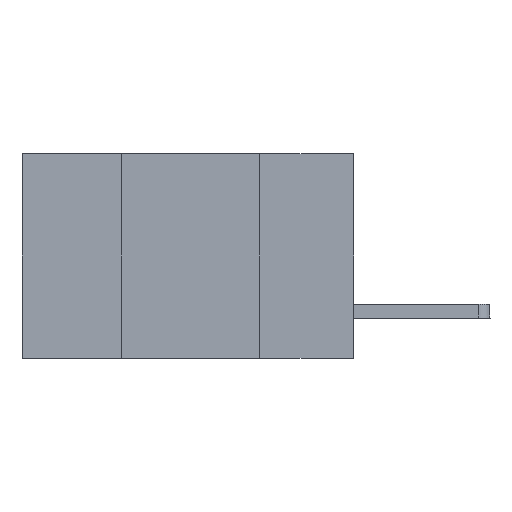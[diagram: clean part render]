
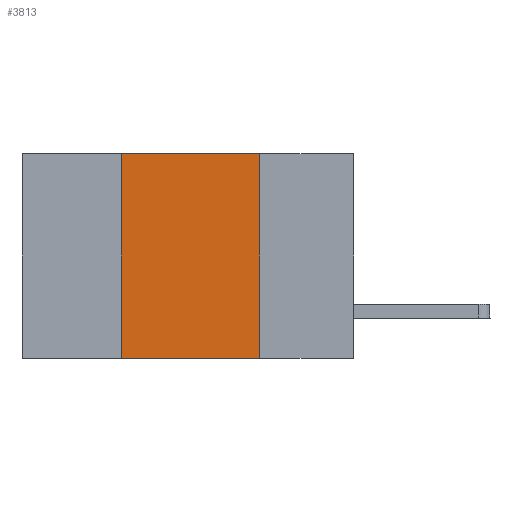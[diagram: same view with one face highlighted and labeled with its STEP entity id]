
A CAD part, left-side view. The second image highlights one B-rep face of the part: STEP entity #3813.
In plain terms, the highlighted planar face has unit normal (-1, 0, 0).
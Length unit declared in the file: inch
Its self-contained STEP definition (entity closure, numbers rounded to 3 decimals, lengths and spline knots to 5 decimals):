
#1851 = EDGE_LOOP ( 'NONE', ( #10755, #11873, #11171, #7456 ) ) ;
#2243 = LINE ( 'NONE', #6458, #7108 ) ;
#2462 = VECTOR ( 'NONE', #10060, 39.37008 ) ;
#2491 = VECTOR ( 'NONE', #9681, 39.37008 ) ;
#2595 = VERTEX_POINT ( 'NONE', #11805 ) ;
#3064 = CARTESIAN_POINT ( 'NONE',  ( 0., 0.6, -0.37 ) ) ;
#3214 = LINE ( 'NONE', #8733, #2491 ) ;
#3367 = DIRECTION ( 'NONE',  ( 0., 0., 1. ) ) ;
#3813 = ADVANCED_FACE ( 'NONE', ( #10261 ), #5046, .F. ) ;
#3956 = VERTEX_POINT ( 'NONE', #11055 ) ;
#4839 = DIRECTION ( 'NONE',  ( 1., 0., 0. ) ) ;
#4885 = DIRECTION ( 'NONE',  ( 0., 0., -1. ) ) ;
#4898 = CARTESIAN_POINT ( 'NONE',  ( 0., 0.6, 0. ) ) ;
#5046 = PLANE ( 'NONE',  #7994 ) ;
#5269 = EDGE_CURVE ( 'NONE', #2595, #11454, #3214, .T. ) ;
#5704 = VECTOR ( 'NONE', #12991, 39.37008 ) ;
#6326 = EDGE_CURVE ( 'NONE', #6690, #3956, #9914, .T. ) ;
#6458 = CARTESIAN_POINT ( 'NONE',  ( 0., 0.42, 0. ) ) ;
#6549 = EDGE_CURVE ( 'NONE', #6690, #2595, #2243, .T. ) ;
#6690 = VERTEX_POINT ( 'NONE', #10481 ) ;
#7108 = VECTOR ( 'NONE', #3367, 39.37008 ) ;
#7456 = ORIENTED_EDGE ( 'NONE', *, *, #6326, .T. ) ;
#7994 = AXIS2_PLACEMENT_3D ( 'NONE', #4898, #4839, #4885 ) ;
#8554 = EDGE_CURVE ( 'NONE', #11454, #3956, #10874, .T. ) ;
#8733 = CARTESIAN_POINT ( 'NONE',  ( 0., 0.6, 0. ) ) ;
#8863 = CARTESIAN_POINT ( 'NONE',  ( 0., 0.17, 0. ) ) ;
#9681 = DIRECTION ( 'NONE',  ( 0., -1., 0. ) ) ;
#9914 = LINE ( 'NONE', #3064, #2462 ) ;
#10060 = DIRECTION ( 'NONE',  ( 0., -1., 0. ) ) ;
#10261 = FACE_OUTER_BOUND ( 'NONE', #1851, .T. ) ;
#10481 = CARTESIAN_POINT ( 'NONE',  ( 0., 0.42, -0.37 ) ) ;
#10755 = ORIENTED_EDGE ( 'NONE', *, *, #8554, .F. ) ;
#10874 = LINE ( 'NONE', #12040, #5704 ) ;
#11055 = CARTESIAN_POINT ( 'NONE',  ( 0., 0.17, -0.37 ) ) ;
#11171 = ORIENTED_EDGE ( 'NONE', *, *, #6549, .F. ) ;
#11454 = VERTEX_POINT ( 'NONE', #8863 ) ;
#11805 = CARTESIAN_POINT ( 'NONE',  ( 0., 0.42, 0. ) ) ;
#11873 = ORIENTED_EDGE ( 'NONE', *, *, #5269, .F. ) ;
#12040 = CARTESIAN_POINT ( 'NONE',  ( 0., 0.17, 0. ) ) ;
#12991 = DIRECTION ( 'NONE',  ( 0., 0., -1. ) ) ;
